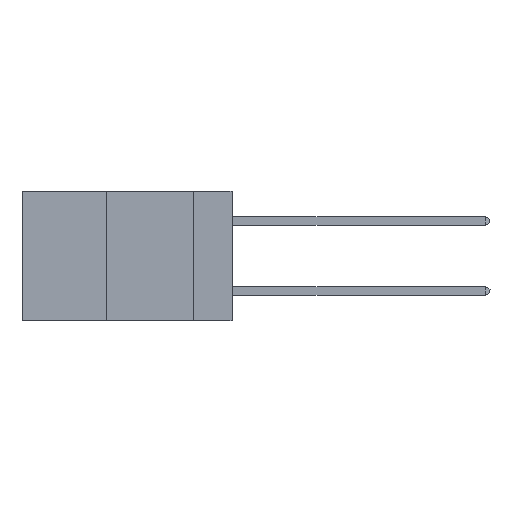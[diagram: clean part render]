
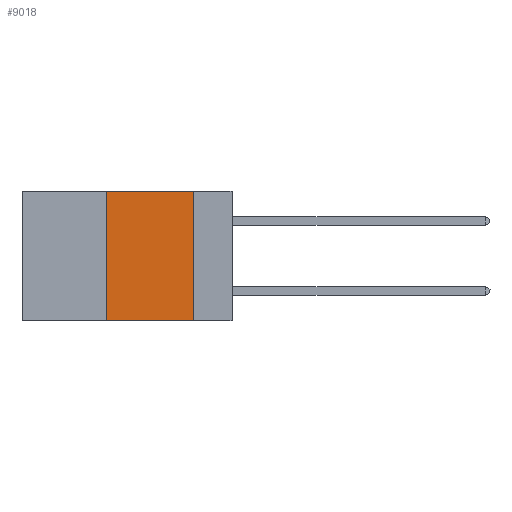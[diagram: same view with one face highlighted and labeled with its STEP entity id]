
A CAD part, left-side view. The second image highlights one B-rep face of the part: STEP entity #9018.
In plain terms, the highlighted planar face has unit normal (-1, 0, 0).
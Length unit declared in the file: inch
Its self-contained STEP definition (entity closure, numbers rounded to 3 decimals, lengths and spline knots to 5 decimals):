
#46 = VECTOR ( 'NONE', #7394, 39.37008 ) ;
#173 = CARTESIAN_POINT ( 'NONE',  ( 0., 0.6, -0.37 ) ) ;
#640 = LINE ( 'NONE', #12687, #8471 ) ;
#647 = ORIENTED_EDGE ( 'NONE', *, *, #6982, .T. ) ;
#867 = EDGE_CURVE ( 'NONE', #6930, #6469, #640, .T. ) ;
#1589 = EDGE_CURVE ( 'NONE', #7063, #14565, #5634, .T. ) ;
#2351 = DIRECTION ( 'NONE',  ( 0., 0., -1. ) ) ;
#3633 = DIRECTION ( 'NONE',  ( 1., 0., 0. ) ) ;
#3960 = DIRECTION ( 'NONE',  ( 0., -1., 0. ) ) ;
#4421 = DIRECTION ( 'NONE',  ( 0., -1., 0. ) ) ;
#5536 = DIRECTION ( 'NONE',  ( 0., 0., 1. ) ) ;
#5634 = LINE ( 'NONE', #5864, #46 ) ;
#5855 = ORIENTED_EDGE ( 'NONE', *, *, #1589, .F. ) ;
#5864 = CARTESIAN_POINT ( 'NONE',  ( 0., 0.11, 0. ) ) ;
#6469 = VERTEX_POINT ( 'NONE', #7251 ) ;
#6716 = LINE ( 'NONE', #173, #12702 ) ;
#6930 = VERTEX_POINT ( 'NONE', #7388 ) ;
#6982 = EDGE_CURVE ( 'NONE', #6930, #14565, #6716, .T. ) ;
#6996 = LINE ( 'NONE', #9251, #13897 ) ;
#7063 = VERTEX_POINT ( 'NONE', #12444 ) ;
#7251 = CARTESIAN_POINT ( 'NONE',  ( 0., 0.36, 0. ) ) ;
#7345 = EDGE_LOOP ( 'NONE', ( #5855, #9164, #9658, #647 ) ) ;
#7388 = CARTESIAN_POINT ( 'NONE',  ( 0., 0.36, -0.37 ) ) ;
#7394 = DIRECTION ( 'NONE',  ( 0., 0., -1. ) ) ;
#8234 = CARTESIAN_POINT ( 'NONE',  ( 0., 0.11, -0.37 ) ) ;
#8471 = VECTOR ( 'NONE', #5536, 39.37008 ) ;
#9018 = ADVANCED_FACE ( 'NONE', ( #9167 ), #9494, .F. ) ;
#9164 = ORIENTED_EDGE ( 'NONE', *, *, #13874, .F. ) ;
#9167 = FACE_OUTER_BOUND ( 'NONE', #7345, .T. ) ;
#9251 = CARTESIAN_POINT ( 'NONE',  ( 0., 0.6, 0. ) ) ;
#9494 = PLANE ( 'NONE',  #11277 ) ;
#9658 = ORIENTED_EDGE ( 'NONE', *, *, #867, .F. ) ;
#11277 = AXIS2_PLACEMENT_3D ( 'NONE', #11963, #3633, #2351 ) ;
#11963 = CARTESIAN_POINT ( 'NONE',  ( 0., 0.6, 0. ) ) ;
#12444 = CARTESIAN_POINT ( 'NONE',  ( 0., 0.11, 0. ) ) ;
#12687 = CARTESIAN_POINT ( 'NONE',  ( 0., 0.36, 0. ) ) ;
#12702 = VECTOR ( 'NONE', #3960, 39.37008 ) ;
#13874 = EDGE_CURVE ( 'NONE', #6469, #7063, #6996, .T. ) ;
#13897 = VECTOR ( 'NONE', #4421, 39.37008 ) ;
#14565 = VERTEX_POINT ( 'NONE', #8234 ) ;
